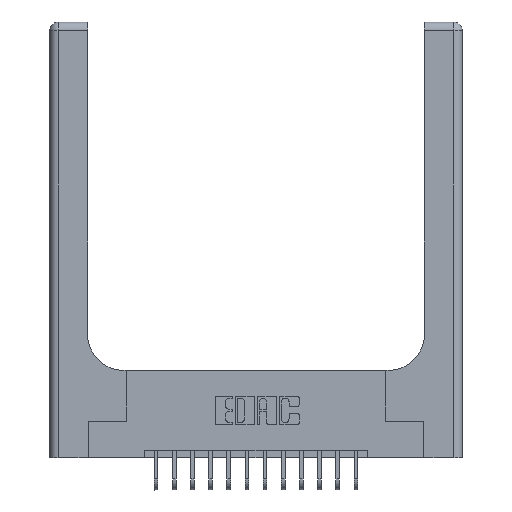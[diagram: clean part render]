
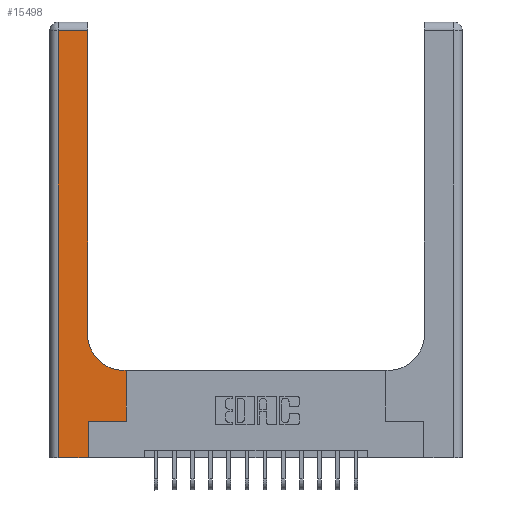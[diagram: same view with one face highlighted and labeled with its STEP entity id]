
A CAD part, top view. The second image highlights one B-rep face of the part: STEP entity #15498.
In plain terms, the highlighted planar face has unit normal (0, 0, 1).
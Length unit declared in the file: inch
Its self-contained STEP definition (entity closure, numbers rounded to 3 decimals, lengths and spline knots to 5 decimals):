
#300 = ORIENTED_EDGE ( 'NONE', *, *, #5761, .T. ) ;
#301 = AXIS2_PLACEMENT_3D ( 'NONE', #10145, #1607, #4500 ) ;
#362 = EDGE_CURVE ( 'NONE', #4249, #8116, #12130, .T. ) ;
#448 = EDGE_CURVE ( 'NONE', #12597, #11929, #3282, .T. ) ;
#859 = VERTEX_POINT ( 'NONE', #9883 ) ;
#1015 = CARTESIAN_POINT ( 'NONE',  ( 0.26, 0.6, 0.37 ) ) ;
#1095 = CARTESIAN_POINT ( 'NONE',  ( 0., 0., 0.37 ) ) ;
#1370 = EDGE_CURVE ( 'NONE', #1396, #13845, #12771, .T. ) ;
#1396 = VERTEX_POINT ( 'NONE', #9853 ) ;
#1454 = EDGE_CURVE ( 'NONE', #859, #4249, #13058, .T. ) ;
#1538 = VERTEX_POINT ( 'NONE', #10424 ) ;
#1607 = DIRECTION ( 'NONE',  ( 0., 0., -1. ) ) ;
#2045 = VECTOR ( 'NONE', #15868, 39.37008 ) ;
#2255 = DIRECTION ( 'NONE',  ( 0., -1., 0. ) ) ;
#2333 = EDGE_CURVE ( 'NONE', #5156, #1396, #14265, .T. ) ;
#2358 = EDGE_CURVE ( 'NONE', #1538, #12597, #10410, .T. ) ;
#2856 = PLANE ( 'NONE',  #301 ) ;
#3282 = LINE ( 'NONE', #1095, #16885 ) ;
#3483 = VECTOR ( 'NONE', #17086, 39.37008 ) ;
#4026 = CARTESIAN_POINT ( 'NONE',  ( 0.26, 3., 0.37 ) ) ;
#4249 = VERTEX_POINT ( 'NONE', #9377 ) ;
#4268 = DIRECTION ( 'NONE',  ( 0., 1., 0. ) ) ;
#4500 = DIRECTION ( 'NONE',  ( -1., 0., 0. ) ) ;
#4577 = CARTESIAN_POINT ( 'NONE',  ( 0.528, 0.6, 0.37 ) ) ;
#4847 = CARTESIAN_POINT ( 'NONE',  ( 0.06, 0., 0.37 ) ) ;
#5021 = DIRECTION ( 'NONE',  ( 0., 0., -1. ) ) ;
#5119 = DIRECTION ( 'NONE',  ( -1., 0., 0. ) ) ;
#5156 = VERTEX_POINT ( 'NONE', #16175 ) ;
#5461 = ORIENTED_EDGE ( 'NONE', *, *, #11331, .T. ) ;
#5761 = EDGE_CURVE ( 'NONE', #8116, #5156, #13900, .T. ) ;
#6751 = LINE ( 'NONE', #11324, #10182 ) ;
#7209 = ORIENTED_EDGE ( 'NONE', *, *, #448, .T. ) ;
#7675 = VECTOR ( 'NONE', #2255, 39.37008 ) ;
#7889 = CARTESIAN_POINT ( 'NONE',  ( 0.06, 3., 0.37 ) ) ;
#8116 = VERTEX_POINT ( 'NONE', #4577 ) ;
#8249 = VECTOR ( 'NONE', #4268, 39.37008 ) ;
#8615 = ORIENTED_EDGE ( 'NONE', *, *, #362, .T. ) ;
#9334 = DIRECTION ( 'NONE',  ( 1., 0., 0. ) ) ;
#9377 = CARTESIAN_POINT ( 'NONE',  ( 0.528, 0.25, 0.37 ) ) ;
#9513 = CARTESIAN_POINT ( 'NONE',  ( 0.51, 0.85, 0.37 ) ) ;
#9853 = CARTESIAN_POINT ( 'NONE',  ( 0.26, 0.85, 0.37 ) ) ;
#9854 = DIRECTION ( 'NONE',  ( 0., 1., 0. ) ) ;
#9883 = CARTESIAN_POINT ( 'NONE',  ( 0.265, 0.25, 0.37 ) ) ;
#10145 = CARTESIAN_POINT ( 'NONE',  ( 0., 3., 0.37 ) ) ;
#10182 = VECTOR ( 'NONE', #9854, 39.37008 ) ;
#10262 = CARTESIAN_POINT ( 'NONE',  ( 0., 2.94, 0.37 ) ) ;
#10410 = LINE ( 'NONE', #7889, #7675 ) ;
#10424 = CARTESIAN_POINT ( 'NONE',  ( 0.06, 2.94, 0.37 ) ) ;
#10593 = AXIS2_PLACEMENT_3D ( 'NONE', #9513, #5021, #9334 ) ;
#10887 = LINE ( 'NONE', #10262, #2045 ) ;
#11324 = CARTESIAN_POINT ( 'NONE',  ( 0.265, 0., 0.37 ) ) ;
#11331 = EDGE_CURVE ( 'NONE', #13845, #1538, #10887, .T. ) ;
#11635 = EDGE_CURVE ( 'NONE', #11929, #859, #6751, .T. ) ;
#11929 = VERTEX_POINT ( 'NONE', #13656 ) ;
#12130 = LINE ( 'NONE', #17265, #8249 ) ;
#12495 = ORIENTED_EDGE ( 'NONE', *, *, #2333, .T. ) ;
#12499 = CARTESIAN_POINT ( 'NONE',  ( 0.26, 2.94, 0.37 ) ) ;
#12597 = VERTEX_POINT ( 'NONE', #4847 ) ;
#12771 = LINE ( 'NONE', #4026, #3483 ) ;
#13058 = LINE ( 'NONE', #14164, #18298 ) ;
#13656 = CARTESIAN_POINT ( 'NONE',  ( 0.265, 0., 0.37 ) ) ;
#13845 = VERTEX_POINT ( 'NONE', #12499 ) ;
#13900 = LINE ( 'NONE', #1015, #18013 ) ;
#13925 = ORIENTED_EDGE ( 'NONE', *, *, #1370, .T. ) ;
#14099 = DIRECTION ( 'NONE',  ( 1., 0., 0. ) ) ;
#14164 = CARTESIAN_POINT ( 'NONE',  ( 0.265, 0.25, 0.37 ) ) ;
#14265 = CIRCLE ( 'NONE', #10593, 0.25 ) ;
#14501 = ORIENTED_EDGE ( 'NONE', *, *, #2358, .T. ) ;
#14723 = ORIENTED_EDGE ( 'NONE', *, *, #11635, .T. ) ;
#15444 = DIRECTION ( 'NONE',  ( 1., 0., 0. ) ) ;
#15498 = ADVANCED_FACE ( 'NONE', ( #17799 ), #2856, .F. ) ;
#15783 = ORIENTED_EDGE ( 'NONE', *, *, #1454, .T. ) ;
#15868 = DIRECTION ( 'NONE',  ( -1., 0., 0. ) ) ;
#16175 = CARTESIAN_POINT ( 'NONE',  ( 0.51, 0.6, 0.37 ) ) ;
#16885 = VECTOR ( 'NONE', #15444, 39.37008 ) ;
#17086 = DIRECTION ( 'NONE',  ( 0., 1., 0. ) ) ;
#17265 = CARTESIAN_POINT ( 'NONE',  ( 0.528, 0.25, 0.37 ) ) ;
#17643 = EDGE_LOOP ( 'NONE', ( #13925, #5461, #14501, #7209, #14723, #15783, #8615, #300, #12495 ) ) ;
#17799 = FACE_OUTER_BOUND ( 'NONE', #17643, .T. ) ;
#18013 = VECTOR ( 'NONE', #5119, 39.37008 ) ;
#18298 = VECTOR ( 'NONE', #14099, 39.37008 ) ;
